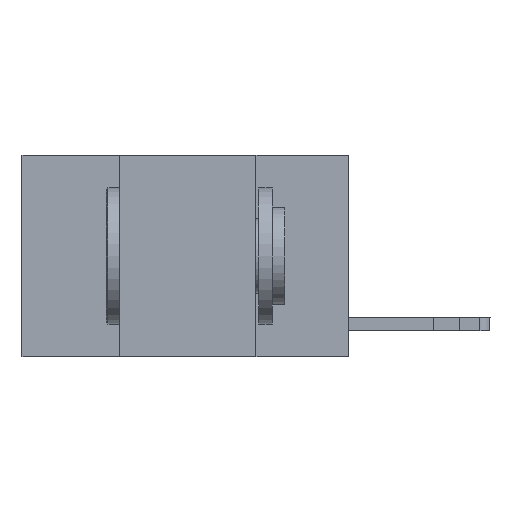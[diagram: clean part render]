
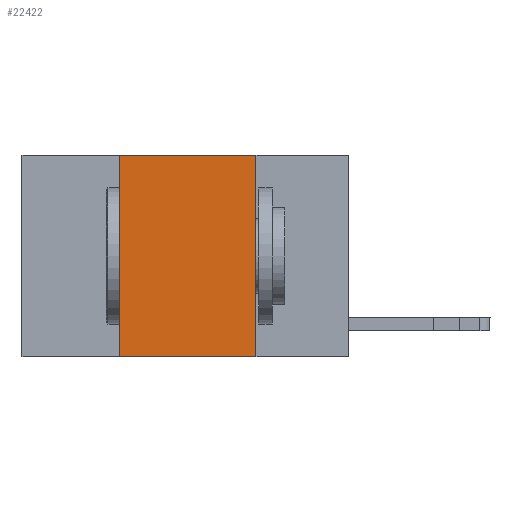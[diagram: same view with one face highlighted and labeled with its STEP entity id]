
A CAD part, left-side view. The second image highlights one B-rep face of the part: STEP entity #22422.
In plain terms, the highlighted planar face has unit normal (-1, 0, 0).
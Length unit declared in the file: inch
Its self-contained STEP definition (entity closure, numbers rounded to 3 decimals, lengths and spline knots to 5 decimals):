
#498 = EDGE_CURVE ( 'NONE', #4457, #2901, #17428, .T. ) ;
#1507 = DIRECTION ( 'NONE',  ( 0., 0., -1. ) ) ;
#1809 = AXIS2_PLACEMENT_3D ( 'NONE', #20012, #12656, #1507 ) ;
#2901 = VERTEX_POINT ( 'NONE', #18017 ) ;
#3197 = VERTEX_POINT ( 'NONE', #13813 ) ;
#3202 = VECTOR ( 'NONE', #6920, 39.37008 ) ;
#4457 = VERTEX_POINT ( 'NONE', #21994 ) ;
#5259 = PLANE ( 'NONE',  #1809 ) ;
#5286 = EDGE_CURVE ( 'NONE', #3197, #17955, #20233, .T. ) ;
#5503 = ORIENTED_EDGE ( 'NONE', *, *, #498, .F. ) ;
#5530 = VECTOR ( 'NONE', #22479, 39.37008 ) ;
#5982 = EDGE_CURVE ( 'NONE', #17955, #4457, #6930, .T. ) ;
#5984 = CARTESIAN_POINT ( 'NONE',  ( 0., 0.42, 0. ) ) ;
#6669 = CARTESIAN_POINT ( 'NONE',  ( 0., 0.17, 0. ) ) ;
#6920 = DIRECTION ( 'NONE',  ( 0., 0., -1. ) ) ;
#6930 = LINE ( 'NONE', #8227, #22144 ) ;
#8227 = CARTESIAN_POINT ( 'NONE',  ( 0., 0.6, 0. ) ) ;
#10389 = ORIENTED_EDGE ( 'NONE', *, *, #5982, .F. ) ;
#10983 = ORIENTED_EDGE ( 'NONE', *, *, #5286, .F. ) ;
#11112 = FACE_OUTER_BOUND ( 'NONE', #19240, .T. ) ;
#11444 = CARTESIAN_POINT ( 'NONE',  ( 0., 0.6, -0.37 ) ) ;
#12656 = DIRECTION ( 'NONE',  ( 1., 0., 0. ) ) ;
#13296 = DIRECTION ( 'NONE',  ( 0., -1., 0. ) ) ;
#13813 = CARTESIAN_POINT ( 'NONE',  ( 0., 0.42, -0.37 ) ) ;
#13973 = LINE ( 'NONE', #11444, #23058 ) ;
#14246 = CARTESIAN_POINT ( 'NONE',  ( 0., 0.42, 0. ) ) ;
#17428 = LINE ( 'NONE', #6669, #3202 ) ;
#17955 = VERTEX_POINT ( 'NONE', #14246 ) ;
#18017 = CARTESIAN_POINT ( 'NONE',  ( 0., 0.17, -0.37 ) ) ;
#19240 = EDGE_LOOP ( 'NONE', ( #5503, #10389, #10983, #20758 ) ) ;
#19668 = EDGE_CURVE ( 'NONE', #3197, #2901, #13973, .T. ) ;
#20012 = CARTESIAN_POINT ( 'NONE',  ( 0., 0.6, 0. ) ) ;
#20233 = LINE ( 'NONE', #5984, #5530 ) ;
#20758 = ORIENTED_EDGE ( 'NONE', *, *, #19668, .T. ) ;
#21994 = CARTESIAN_POINT ( 'NONE',  ( 0., 0.17, 0. ) ) ;
#22144 = VECTOR ( 'NONE', #22831, 39.37008 ) ;
#22422 = ADVANCED_FACE ( 'NONE', ( #11112 ), #5259, .F. ) ;
#22479 = DIRECTION ( 'NONE',  ( 0., 0., 1. ) ) ;
#22831 = DIRECTION ( 'NONE',  ( 0., -1., 0. ) ) ;
#23058 = VECTOR ( 'NONE', #13296, 39.37008 ) ;
